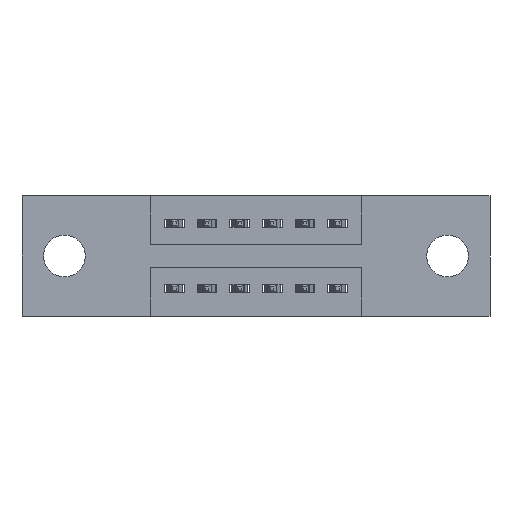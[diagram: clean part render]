
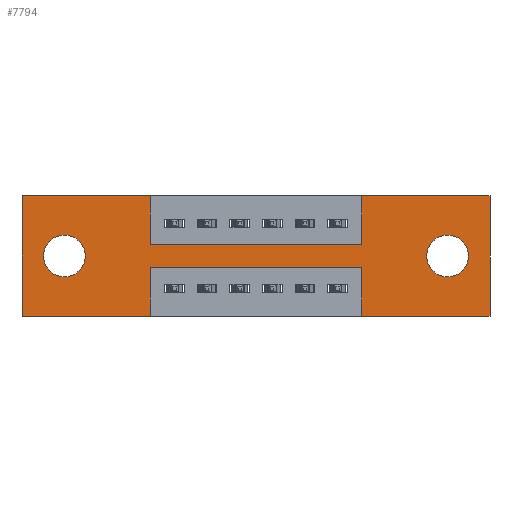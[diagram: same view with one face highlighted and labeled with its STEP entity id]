
A CAD part, front view. The second image highlights one B-rep face of the part: STEP entity #7794.
In plain terms, the highlighted planar face has unit normal (0, -1, 0).
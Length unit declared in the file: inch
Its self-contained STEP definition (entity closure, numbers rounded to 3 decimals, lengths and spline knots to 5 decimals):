
#20 = LINE ( 'NONE', #7574, #7658 ) ;
#100 = VERTEX_POINT ( 'NONE', #3674 ) ;
#115 = ORIENTED_EDGE ( 'NONE', *, *, #1699, .F. ) ;
#167 = VERTEX_POINT ( 'NONE', #4582 ) ;
#263 = ORIENTED_EDGE ( 'NONE', *, *, #6733, .F. ) ;
#732 = VERTEX_POINT ( 'NONE', #1272 ) ;
#812 = CARTESIAN_POINT ( 'NONE',  ( 1.0425, 0., -0.22 ) ) ;
#830 = ORIENTED_EDGE ( 'NONE', *, *, #2291, .F. ) ;
#878 = DIRECTION ( 'NONE',  ( -1., 0., 0. ) ) ;
#934 = AXIS2_PLACEMENT_3D ( 'NONE', #1573, #6789, #2327 ) ;
#964 = VECTOR ( 'NONE', #7164, 39.37008 ) ;
#1146 = CARTESIAN_POINT ( 'NONE',  ( 1.0425, 0., -0.37 ) ) ;
#1197 = ORIENTED_EDGE ( 'NONE', *, *, #5756, .F. ) ;
#1207 = AXIS2_PLACEMENT_3D ( 'NONE', #2298, #4566, #3840 ) ;
#1272 = CARTESIAN_POINT ( 'NONE',  ( 0.3925, 0., -0.15 ) ) ;
#1274 = FACE_BOUND ( 'NONE', #3053, .T. ) ;
#1327 = VERTEX_POINT ( 'NONE', #5824 ) ;
#1377 = VECTOR ( 'NONE', #4214, 39.37008 ) ;
#1573 = CARTESIAN_POINT ( 'NONE',  ( 1.305, 0., -0.185 ) ) ;
#1597 = FACE_BOUND ( 'NONE', #7681, .T. ) ;
#1635 = ORIENTED_EDGE ( 'NONE', *, *, #5293, .F. ) ;
#1690 = DIRECTION ( 'NONE',  ( 0., 0., 1. ) ) ;
#1699 = EDGE_CURVE ( 'NONE', #6593, #9177, #2027, .T. ) ;
#1984 = CARTESIAN_POINT ( 'NONE',  ( 0.3925, 0., -0.22 ) ) ;
#2027 = LINE ( 'NONE', #7532, #4764 ) ;
#2058 = ORIENTED_EDGE ( 'NONE', *, *, #5056, .F. ) ;
#2105 = ORIENTED_EDGE ( 'NONE', *, *, #7736, .T. ) ;
#2178 = EDGE_CURVE ( 'NONE', #5427, #9283, #6460, .T. ) ;
#2188 = VERTEX_POINT ( 'NONE', #812 ) ;
#2206 = DIRECTION ( 'NONE',  ( -1., 0., 0. ) ) ;
#2291 = EDGE_CURVE ( 'NONE', #732, #1327, #6349, .T. ) ;
#2298 = CARTESIAN_POINT ( 'NONE',  ( 1.305, 0., -0.185 ) ) ;
#2327 = DIRECTION ( 'NONE',  ( 0., 0., -1. ) ) ;
#2434 = CARTESIAN_POINT ( 'NONE',  ( 0.3925, 0., -0.22 ) ) ;
#2466 = ORIENTED_EDGE ( 'NONE', *, *, #8880, .T. ) ;
#2587 = EDGE_CURVE ( 'NONE', #5382, #3538, #5086, .T. ) ;
#2629 = CARTESIAN_POINT ( 'NONE',  ( 0., 0., 0. ) ) ;
#2754 = VERTEX_POINT ( 'NONE', #1984 ) ;
#2901 = CARTESIAN_POINT ( 'NONE',  ( 0., 0., -0.37 ) ) ;
#2953 = DIRECTION ( 'NONE',  ( 0., 0., 1. ) ) ;
#3053 = EDGE_LOOP ( 'NONE', ( #7038, #2105 ) ) ;
#3069 = CARTESIAN_POINT ( 'NONE',  ( 0.3925, 0., 0. ) ) ;
#3120 = CARTESIAN_POINT ( 'NONE',  ( 0., 0., -0.37 ) ) ;
#3194 = VECTOR ( 'NONE', #5676, 39.37008 ) ;
#3211 = CARTESIAN_POINT ( 'NONE',  ( 0.13, 0., -0.121 ) ) ;
#3281 = LINE ( 'NONE', #4241, #3998 ) ;
#3355 = CARTESIAN_POINT ( 'NONE',  ( 0.3925, 0., -0.15 ) ) ;
#3378 = ORIENTED_EDGE ( 'NONE', *, *, #3611, .F. ) ;
#3406 = CARTESIAN_POINT ( 'NONE',  ( 1.0425, 0., -0.37 ) ) ;
#3438 = ORIENTED_EDGE ( 'NONE', *, *, #2587, .F. ) ;
#3538 = VERTEX_POINT ( 'NONE', #5605 ) ;
#3604 = CIRCLE ( 'NONE', #9263, 0.064 ) ;
#3611 = EDGE_CURVE ( 'NONE', #2754, #8637, #3901, .T. ) ;
#3674 = CARTESIAN_POINT ( 'NONE',  ( 0.13, 0., -0.249 ) ) ;
#3733 = EDGE_CURVE ( 'NONE', #4938, #100, #3897, .T. ) ;
#3840 = DIRECTION ( 'NONE',  ( 0., 0., -1. ) ) ;
#3857 = VERTEX_POINT ( 'NONE', #1146 ) ;
#3897 = CIRCLE ( 'NONE', #5665, 0.064 ) ;
#3901 = LINE ( 'NONE', #5260, #4134 ) ;
#3927 = EDGE_CURVE ( 'NONE', #3857, #2188, #7558, .T. ) ;
#3998 = VECTOR ( 'NONE', #5348, 39.37008 ) ;
#4134 = VECTOR ( 'NONE', #4436, 39.37008 ) ;
#4214 = DIRECTION ( 'NONE',  ( 1., 0., 0. ) ) ;
#4241 = CARTESIAN_POINT ( 'NONE',  ( 0.3925, 0., 0. ) ) ;
#4316 = ORIENTED_EDGE ( 'NONE', *, *, #6650, .F. ) ;
#4372 = EDGE_CURVE ( 'NONE', #7525, #732, #3281, .T. ) ;
#4436 = DIRECTION ( 'NONE',  ( 0., 0., -1. ) ) ;
#4546 = VECTOR ( 'NONE', #8340, 39.37008 ) ;
#4550 = PLANE ( 'NONE',  #7632 ) ;
#4566 = DIRECTION ( 'NONE',  ( 0., 1., 0. ) ) ;
#4582 = CARTESIAN_POINT ( 'NONE',  ( 1.0425, 0., 0. ) ) ;
#4693 = LINE ( 'NONE', #6242, #1377 ) ;
#4694 = DIRECTION ( 'NONE',  ( 0., -1., 0. ) ) ;
#4708 = CARTESIAN_POINT ( 'NONE',  ( 1.305, 0., -0.121 ) ) ;
#4709 = DIRECTION ( 'NONE',  ( 0., 1., 0. ) ) ;
#4720 = VECTOR ( 'NONE', #5720, 39.37008 ) ;
#4764 = VECTOR ( 'NONE', #9068, 39.37008 ) ;
#4916 = ORIENTED_EDGE ( 'NONE', *, *, #7109, .F. ) ;
#4938 = VERTEX_POINT ( 'NONE', #3211 ) ;
#4957 = ORIENTED_EDGE ( 'NONE', *, *, #2178, .T. ) ;
#4973 = CARTESIAN_POINT ( 'NONE',  ( 0.3925, 0., -0.37 ) ) ;
#5056 = EDGE_CURVE ( 'NONE', #9177, #7525, #4693, .T. ) ;
#5086 = LINE ( 'NONE', #7934, #964 ) ;
#5098 = ORIENTED_EDGE ( 'NONE', *, *, #4372, .F. ) ;
#5259 = CARTESIAN_POINT ( 'NONE',  ( 0., 0., 0. ) ) ;
#5260 = CARTESIAN_POINT ( 'NONE',  ( 0.3925, 0., -0.37 ) ) ;
#5293 = EDGE_CURVE ( 'NONE', #167, #5382, #8923, .T. ) ;
#5338 = DIRECTION ( 'NONE',  ( 0., 0., 1. ) ) ;
#5348 = DIRECTION ( 'NONE',  ( 0., 0., -1. ) ) ;
#5382 = VERTEX_POINT ( 'NONE', #6131 ) ;
#5427 = VERTEX_POINT ( 'NONE', #4708 ) ;
#5531 = CARTESIAN_POINT ( 'NONE',  ( 0., 0., -0.37 ) ) ;
#5605 = CARTESIAN_POINT ( 'NONE',  ( 1.435, 0., -0.37 ) ) ;
#5665 = AXIS2_PLACEMENT_3D ( 'NONE', #7620, #4709, #1690 ) ;
#5676 = DIRECTION ( 'NONE',  ( 1., 0., 0. ) ) ;
#5720 = DIRECTION ( 'NONE',  ( 0., 0., 1. ) ) ;
#5756 = EDGE_CURVE ( 'NONE', #8637, #6593, #7731, .T. ) ;
#5824 = CARTESIAN_POINT ( 'NONE',  ( 1.0425, 0., -0.15 ) ) ;
#5907 = DIRECTION ( 'NONE',  ( 1., 0., 0. ) ) ;
#6082 = LINE ( 'NONE', #6553, #9516 ) ;
#6131 = CARTESIAN_POINT ( 'NONE',  ( 1.435, 0., 0. ) ) ;
#6242 = CARTESIAN_POINT ( 'NONE',  ( 0., 0., 0. ) ) ;
#6268 = CIRCLE ( 'NONE', #934, 0.064 ) ;
#6340 = CARTESIAN_POINT ( 'NONE',  ( 0.13, 0., -0.185 ) ) ;
#6349 = LINE ( 'NONE', #3355, #3194 ) ;
#6460 = CIRCLE ( 'NONE', #1207, 0.064 ) ;
#6553 = CARTESIAN_POINT ( 'NONE',  ( 0., 0., -0.37 ) ) ;
#6593 = VERTEX_POINT ( 'NONE', #2901 ) ;
#6650 = EDGE_CURVE ( 'NONE', #3538, #3857, #6082, .T. ) ;
#6733 = EDGE_CURVE ( 'NONE', #1327, #167, #20, .T. ) ;
#6789 = DIRECTION ( 'NONE',  ( 0., 1., 0. ) ) ;
#6811 = DIRECTION ( 'NONE',  ( 0., 1., 0. ) ) ;
#6952 = VECTOR ( 'NONE', #5907, 39.37008 ) ;
#7038 = ORIENTED_EDGE ( 'NONE', *, *, #3733, .T. ) ;
#7109 = EDGE_CURVE ( 'NONE', #2188, #2754, #9174, .T. ) ;
#7110 = DIRECTION ( 'NONE',  ( 0., 0., -1. ) ) ;
#7164 = DIRECTION ( 'NONE',  ( 0., 0., -1. ) ) ;
#7429 = ORIENTED_EDGE ( 'NONE', *, *, #3927, .F. ) ;
#7525 = VERTEX_POINT ( 'NONE', #3069 ) ;
#7532 = CARTESIAN_POINT ( 'NONE',  ( 0., 0., 0. ) ) ;
#7558 = LINE ( 'NONE', #3406, #4720 ) ;
#7574 = CARTESIAN_POINT ( 'NONE',  ( 1.0425, 0., 0. ) ) ;
#7620 = CARTESIAN_POINT ( 'NONE',  ( 0.13, 0., -0.185 ) ) ;
#7632 = AXIS2_PLACEMENT_3D ( 'NONE', #3120, #4694, #7110 ) ;
#7658 = VECTOR ( 'NONE', #5338, 39.37008 ) ;
#7681 = EDGE_LOOP ( 'NONE', ( #4957, #2466 ) ) ;
#7731 = LINE ( 'NONE', #5531, #4546 ) ;
#7736 = EDGE_CURVE ( 'NONE', #100, #4938, #3604, .T. ) ;
#7794 = ADVANCED_FACE ( 'NONE', ( #1597, #1274, #8928 ), #4550, .T. ) ;
#7934 = CARTESIAN_POINT ( 'NONE',  ( 1.435, 0., 0. ) ) ;
#8340 = DIRECTION ( 'NONE',  ( -1., 0., 0. ) ) ;
#8565 = CARTESIAN_POINT ( 'NONE',  ( 1.305, 0., -0.249 ) ) ;
#8637 = VERTEX_POINT ( 'NONE', #4973 ) ;
#8836 = VECTOR ( 'NONE', #878, 39.37008 ) ;
#8880 = EDGE_CURVE ( 'NONE', #9283, #5427, #6268, .T. ) ;
#8923 = LINE ( 'NONE', #5259, #6952 ) ;
#8928 = FACE_OUTER_BOUND ( 'NONE', #9396, .T. ) ;
#9068 = DIRECTION ( 'NONE',  ( 0., 0., 1. ) ) ;
#9174 = LINE ( 'NONE', #2434, #8836 ) ;
#9177 = VERTEX_POINT ( 'NONE', #2629 ) ;
#9263 = AXIS2_PLACEMENT_3D ( 'NONE', #6340, #6811, #2953 ) ;
#9283 = VERTEX_POINT ( 'NONE', #8565 ) ;
#9396 = EDGE_LOOP ( 'NONE', ( #3378, #4916, #7429, #4316, #3438, #1635, #263, #830, #5098, #2058, #115, #1197 ) ) ;
#9516 = VECTOR ( 'NONE', #2206, 39.37008 ) ;
